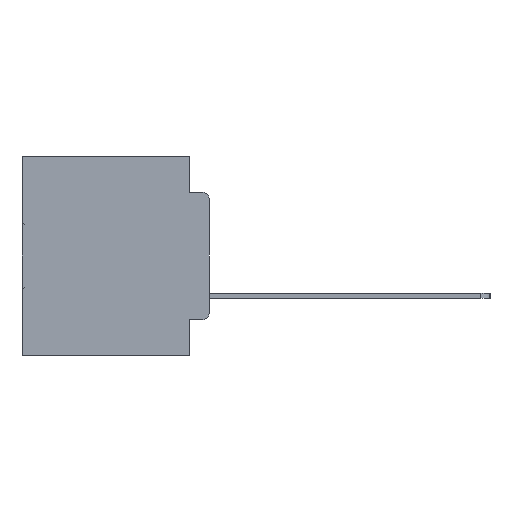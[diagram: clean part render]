
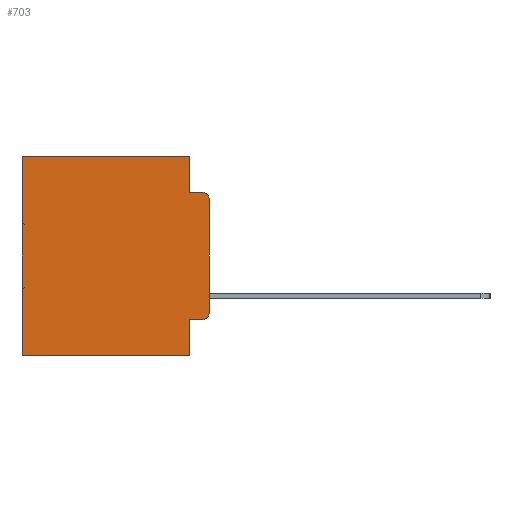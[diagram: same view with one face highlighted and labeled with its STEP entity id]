
A CAD part, left-side view. The second image highlights one B-rep face of the part: STEP entity #703.
In plain terms, the highlighted planar face has unit normal (-1, 0, 0).
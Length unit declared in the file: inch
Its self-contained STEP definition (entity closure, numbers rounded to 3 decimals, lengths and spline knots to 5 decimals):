
#58 = VECTOR ( 'NONE', #21161, 39.37008 ) ;
#703 = ADVANCED_FACE ( 'NONE', ( #20889 ), #20256, .F. ) ;
#2029 = AXIS2_PLACEMENT_3D ( 'NONE', #16976, #20450, #3266 ) ;
#2114 = DIRECTION ( 'NONE',  ( -1., 0., 0. ) ) ;
#2525 = VERTEX_POINT ( 'NONE', #17015 ) ;
#2668 = VERTEX_POINT ( 'NONE', #13657 ) ;
#2751 = CARTESIAN_POINT ( 'NONE',  ( 0.298, 0.02, -0.3915 ) ) ;
#3026 = ORIENTED_EDGE ( 'NONE', *, *, #31273, .T. ) ;
#3266 = DIRECTION ( 'NONE',  ( 0., 0., -1. ) ) ;
#4144 = ORIENTED_EDGE ( 'NONE', *, *, #13697, .T. ) ;
#4845 = DIRECTION ( 'NONE',  ( 0., 0., -1. ) ) ;
#5155 = VERTEX_POINT ( 'NONE', #11690 ) ;
#5375 = CARTESIAN_POINT ( 'NONE',  ( 0.298, 0.051, -0.4115 ) ) ;
#5413 = DIRECTION ( 'NONE',  ( 0., 0., -1. ) ) ;
#5439 = LINE ( 'NONE', #13759, #11626 ) ;
#5521 = CIRCLE ( 'NONE', #20678, 0.02 ) ;
#5686 = LINE ( 'NONE', #26986, #11893 ) ;
#6031 = EDGE_CURVE ( 'NONE', #27977, #2668, #28108, .T. ) ;
#6683 = EDGE_CURVE ( 'NONE', #2525, #14861, #28456, .T. ) ;
#6843 = CARTESIAN_POINT ( 'NONE',  ( 0.298, 0.02, -0.4115 ) ) ;
#7730 = VECTOR ( 'NONE', #4845, 39.37008 ) ;
#7846 = VECTOR ( 'NONE', #16561, 39.37008 ) ;
#8124 = AXIS2_PLACEMENT_3D ( 'NONE', #17704, #2114, #20265 ) ;
#8624 = LINE ( 'NONE', #24661, #33251 ) ;
#10750 = VERTEX_POINT ( 'NONE', #20391 ) ;
#11196 = LINE ( 'NONE', #19032, #23122 ) ;
#11626 = VECTOR ( 'NONE', #28892, 39.37008 ) ;
#11690 = CARTESIAN_POINT ( 'NONE',  ( 0.298, 0.473, -0.5 ) ) ;
#11716 = ORIENTED_EDGE ( 'NONE', *, *, #25596, .F. ) ;
#11893 = VECTOR ( 'NONE', #29499, 39.37008 ) ;
#12008 = EDGE_CURVE ( 'NONE', #2525, #15685, #5439, .T. ) ;
#12779 = CARTESIAN_POINT ( 'NONE',  ( 0.298, 0., 0. ) ) ;
#13657 = CARTESIAN_POINT ( 'NONE',  ( 0.298, 0., -0.3915 ) ) ;
#13697 = EDGE_CURVE ( 'NONE', #26838, #5155, #8624, .T. ) ;
#13759 = CARTESIAN_POINT ( 'NONE',  ( 0.298, 0.051, 0. ) ) ;
#13987 = CARTESIAN_POINT ( 'NONE',  ( 0.298, 0., 0. ) ) ;
#14831 = CARTESIAN_POINT ( 'NONE',  ( 0.298, 0.051, 0. ) ) ;
#14861 = VERTEX_POINT ( 'NONE', #6843 ) ;
#14927 = ORIENTED_EDGE ( 'NONE', *, *, #33189, .F. ) ;
#15685 = VERTEX_POINT ( 'NONE', #25427 ) ;
#15721 = DIRECTION ( 'NONE',  ( 0., -1., 0. ) ) ;
#16561 = DIRECTION ( 'NONE',  ( 0., 1., 0. ) ) ;
#16586 = DIRECTION ( 'NONE',  ( 0., 0., -1. ) ) ;
#16682 = CIRCLE ( 'NONE', #8124, 0.02 ) ;
#16976 = CARTESIAN_POINT ( 'NONE',  ( 0.298, 0., 0. ) ) ;
#17015 = CARTESIAN_POINT ( 'NONE',  ( 0.298, 0.051, -0.4115 ) ) ;
#17313 = ORIENTED_EDGE ( 'NONE', *, *, #28945, .T. ) ;
#17698 = ORIENTED_EDGE ( 'NONE', *, *, #23917, .F. ) ;
#17704 = CARTESIAN_POINT ( 'NONE',  ( 0.298, 0.02, -0.1085 ) ) ;
#17880 = VERTEX_POINT ( 'NONE', #14831 ) ;
#18656 = CARTESIAN_POINT ( 'NONE',  ( 0.298, 0., -0.5 ) ) ;
#19032 = CARTESIAN_POINT ( 'NONE',  ( 0.298, 0.051, 0. ) ) ;
#20256 = PLANE ( 'NONE',  #2029 ) ;
#20265 = DIRECTION ( 'NONE',  ( 0., 0., -1. ) ) ;
#20391 = CARTESIAN_POINT ( 'NONE',  ( 0.298, 0.051, -0.0885 ) ) ;
#20450 = DIRECTION ( 'NONE',  ( 1., 0., 0. ) ) ;
#20678 = AXIS2_PLACEMENT_3D ( 'NONE', #2751, #20858, #5413 ) ;
#20781 = LINE ( 'NONE', #18656, #58 ) ;
#20858 = DIRECTION ( 'NONE',  ( -1., 0., 0. ) ) ;
#20889 = FACE_OUTER_BOUND ( 'NONE', #23039, .T. ) ;
#21161 = DIRECTION ( 'NONE',  ( 0., 1., 0. ) ) ;
#21580 = ORIENTED_EDGE ( 'NONE', *, *, #12008, .F. ) ;
#21794 = ORIENTED_EDGE ( 'NONE', *, *, #6031, .F. ) ;
#23039 = EDGE_LOOP ( 'NONE', ( #21794, #17313, #11716, #17698, #27959, #4144, #14927, #21580, #23625, #3026 ) ) ;
#23122 = VECTOR ( 'NONE', #16586, 39.37008 ) ;
#23625 = ORIENTED_EDGE ( 'NONE', *, *, #6683, .T. ) ;
#23917 = EDGE_CURVE ( 'NONE', #17880, #10750, #11196, .T. ) ;
#24386 = EDGE_CURVE ( 'NONE', #17880, #26838, #28225, .T. ) ;
#24492 = CARTESIAN_POINT ( 'NONE',  ( 0.298, 0.473, 0. ) ) ;
#24661 = CARTESIAN_POINT ( 'NONE',  ( 0.298, 0.473, 0. ) ) ;
#25427 = CARTESIAN_POINT ( 'NONE',  ( 0.298, 0.051, -0.5 ) ) ;
#25596 = EDGE_CURVE ( 'NONE', #10750, #32024, #5686, .T. ) ;
#25936 = CARTESIAN_POINT ( 'NONE',  ( 0.298, 0., -0.1085 ) ) ;
#26838 = VERTEX_POINT ( 'NONE', #24492 ) ;
#26986 = CARTESIAN_POINT ( 'NONE',  ( 0.298, 0.051, -0.0885 ) ) ;
#27170 = DIRECTION ( 'NONE',  ( 0., 0., -1. ) ) ;
#27671 = VECTOR ( 'NONE', #15721, 39.37008 ) ;
#27959 = ORIENTED_EDGE ( 'NONE', *, *, #24386, .T. ) ;
#27977 = VERTEX_POINT ( 'NONE', #25936 ) ;
#28108 = LINE ( 'NONE', #12779, #7730 ) ;
#28225 = LINE ( 'NONE', #13987, #7846 ) ;
#28456 = LINE ( 'NONE', #5375, #27671 ) ;
#28892 = DIRECTION ( 'NONE',  ( 0., 0., -1. ) ) ;
#28945 = EDGE_CURVE ( 'NONE', #27977, #32024, #16682, .T. ) ;
#29063 = CARTESIAN_POINT ( 'NONE',  ( 0.298, 0.02, -0.0885 ) ) ;
#29499 = DIRECTION ( 'NONE',  ( 0., -1., 0. ) ) ;
#31273 = EDGE_CURVE ( 'NONE', #14861, #2668, #5521, .T. ) ;
#32024 = VERTEX_POINT ( 'NONE', #29063 ) ;
#33189 = EDGE_CURVE ( 'NONE', #15685, #5155, #20781, .T. ) ;
#33251 = VECTOR ( 'NONE', #27170, 39.37008 ) ;
